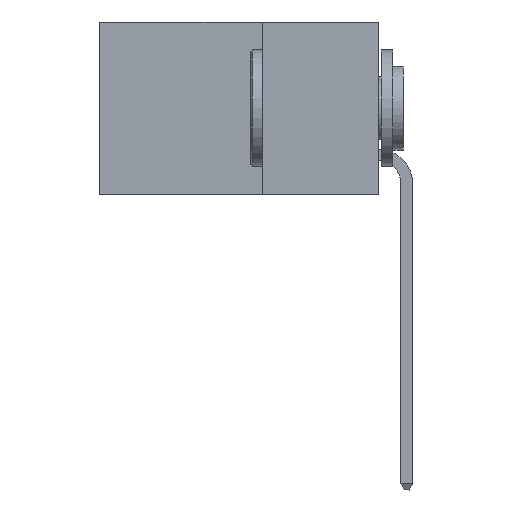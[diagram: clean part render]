
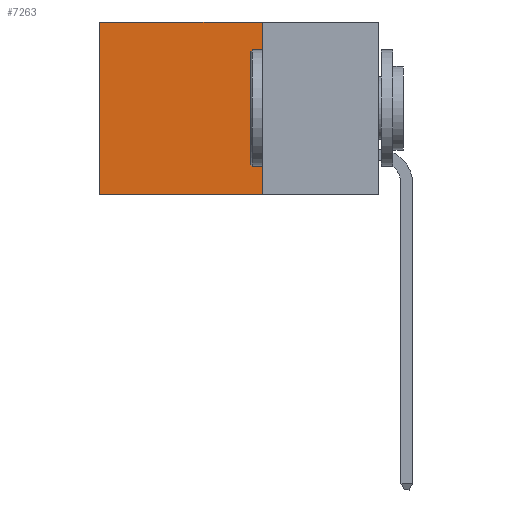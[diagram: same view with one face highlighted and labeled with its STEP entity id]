
A CAD part, left-side view. The second image highlights one B-rep face of the part: STEP entity #7263.
In plain terms, the highlighted planar face has unit normal (-1, 0, 0).
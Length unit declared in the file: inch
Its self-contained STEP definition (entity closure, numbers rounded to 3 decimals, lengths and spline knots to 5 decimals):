
#1043 = DIRECTION ( 'NONE',  ( 0., 0., -1. ) ) ;
#2815 = EDGE_LOOP ( 'NONE', ( #24591, #3949, #12652, #15441 ) ) ;
#3300 = DIRECTION ( 'NONE',  ( 0., 1., 0. ) ) ;
#3949 = ORIENTED_EDGE ( 'NONE', *, *, #8216, .F. ) ;
#4655 = EDGE_CURVE ( 'NONE', #14910, #10543, #24256, .T. ) ;
#7263 = ADVANCED_FACE ( 'NONE', ( #9003 ), #18454, .F. ) ;
#7698 = CARTESIAN_POINT ( 'NONE',  ( 0.298, 0.25, 0. ) ) ;
#7931 = DIRECTION ( 'NONE',  ( 0., 1., 0. ) ) ;
#8216 = EDGE_CURVE ( 'NONE', #17315, #10543, #15513, .T. ) ;
#8898 = CARTESIAN_POINT ( 'NONE',  ( 0.298, 0.6, -0.37 ) ) ;
#8950 = DIRECTION ( 'NONE',  ( 0., 0., -1. ) ) ;
#9003 = FACE_OUTER_BOUND ( 'NONE', #2815, .T. ) ;
#9115 = VECTOR ( 'NONE', #1043, 39.37008 ) ;
#9852 = VECTOR ( 'NONE', #7931, 39.37008 ) ;
#10543 = VERTEX_POINT ( 'NONE', #8898 ) ;
#10611 = LINE ( 'NONE', #15672, #18956 ) ;
#12652 = ORIENTED_EDGE ( 'NONE', *, *, #23825, .F. ) ;
#13478 = CARTESIAN_POINT ( 'NONE',  ( 0.298, 0.6, 0. ) ) ;
#13572 = CARTESIAN_POINT ( 'NONE',  ( 0.298, 0.25, -0.37 ) ) ;
#14223 = VERTEX_POINT ( 'NONE', #7698 ) ;
#14363 = CARTESIAN_POINT ( 'NONE',  ( 0.298, 0.6, 0. ) ) ;
#14684 = LINE ( 'NONE', #18541, #19141 ) ;
#14910 = VERTEX_POINT ( 'NONE', #13478 ) ;
#15441 = ORIENTED_EDGE ( 'NONE', *, *, #16336, .T. ) ;
#15513 = LINE ( 'NONE', #13572, #9852 ) ;
#15672 = CARTESIAN_POINT ( 'NONE',  ( 0.298, 0.25, 0. ) ) ;
#16336 = EDGE_CURVE ( 'NONE', #14223, #14910, #14684, .T. ) ;
#16539 = CARTESIAN_POINT ( 'NONE',  ( 0.298, 0.25, 0. ) ) ;
#17315 = VERTEX_POINT ( 'NONE', #21558 ) ;
#17606 = DIRECTION ( 'NONE',  ( 0., 0., -1. ) ) ;
#18454 = PLANE ( 'NONE',  #19717 ) ;
#18541 = CARTESIAN_POINT ( 'NONE',  ( 0.298, 0.25, 0. ) ) ;
#18956 = VECTOR ( 'NONE', #17606, 39.37008 ) ;
#19141 = VECTOR ( 'NONE', #3300, 39.37008 ) ;
#19717 = AXIS2_PLACEMENT_3D ( 'NONE', #16539, #20333, #8950 ) ;
#20333 = DIRECTION ( 'NONE',  ( 1., 0., 0. ) ) ;
#21558 = CARTESIAN_POINT ( 'NONE',  ( 0.298, 0.25, -0.37 ) ) ;
#23825 = EDGE_CURVE ( 'NONE', #14223, #17315, #10611, .T. ) ;
#24256 = LINE ( 'NONE', #14363, #9115 ) ;
#24591 = ORIENTED_EDGE ( 'NONE', *, *, #4655, .T. ) ;
